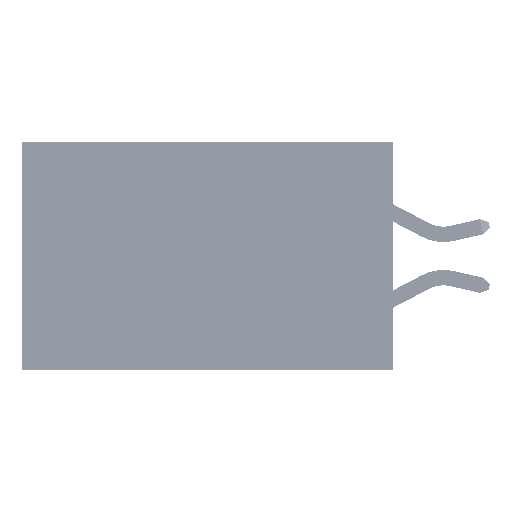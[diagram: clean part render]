
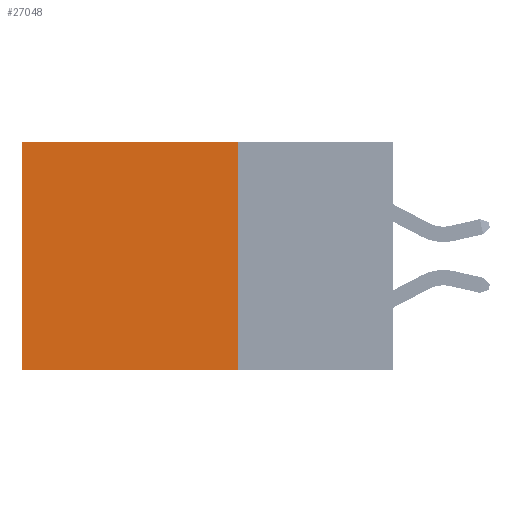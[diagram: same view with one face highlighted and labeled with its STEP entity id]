
A CAD part, left-side view. The second image highlights one B-rep face of the part: STEP entity #27048.
In plain terms, the highlighted planar face has unit normal (-1, 0, 0).
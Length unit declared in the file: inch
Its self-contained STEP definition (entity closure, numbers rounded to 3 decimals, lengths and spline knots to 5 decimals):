
#1830 = ORIENTED_EDGE ( 'NONE', *, *, #5780, .T. ) ;
#2251 = AXIS2_PLACEMENT_3D ( 'NONE', #22055, #33531, #18820 ) ;
#2702 = FACE_OUTER_BOUND ( 'NONE', #6475, .T. ) ;
#5780 = EDGE_CURVE ( 'NONE', #14651, #26979, #20097, .T. ) ;
#6475 = EDGE_LOOP ( 'NONE', ( #14346, #16748, #8131, #1830 ) ) ;
#8131 = ORIENTED_EDGE ( 'NONE', *, *, #28855, .F. ) ;
#9143 = VECTOR ( 'NONE', #19988, 39.37008 ) ;
#9574 = LINE ( 'NONE', #16689, #29916 ) ;
#12429 = VERTEX_POINT ( 'NONE', #32732 ) ;
#14346 = ORIENTED_EDGE ( 'NONE', *, *, #26588, .T. ) ;
#14651 = VERTEX_POINT ( 'NONE', #32349 ) ;
#15039 = CARTESIAN_POINT ( 'NONE',  ( 0.2875, 0.6, 0. ) ) ;
#16535 = VECTOR ( 'NONE', #17189, 39.37008 ) ;
#16689 = CARTESIAN_POINT ( 'NONE',  ( 0.2875, 0.25, -0.37 ) ) ;
#16748 = ORIENTED_EDGE ( 'NONE', *, *, #21354, .F. ) ;
#16850 = DIRECTION ( 'NONE',  ( 0., 1., 0. ) ) ;
#17189 = DIRECTION ( 'NONE',  ( 0., 0., -1. ) ) ;
#18820 = DIRECTION ( 'NONE',  ( 0., 0., -1. ) ) ;
#19988 = DIRECTION ( 'NONE',  ( 0., 0., -1. ) ) ;
#20097 = LINE ( 'NONE', #20265, #47301 ) ;
#20265 = CARTESIAN_POINT ( 'NONE',  ( 0.2875, 0.25, 0. ) ) ;
#21354 = EDGE_CURVE ( 'NONE', #12429, #30781, #9574, .T. ) ;
#22055 = CARTESIAN_POINT ( 'NONE',  ( 0.2875, 0.25, 0. ) ) ;
#23180 = DIRECTION ( 'NONE',  ( 0., 1., 0. ) ) ;
#26588 = EDGE_CURVE ( 'NONE', #26979, #30781, #41065, .T. ) ;
#26979 = VERTEX_POINT ( 'NONE', #15039 ) ;
#27048 = ADVANCED_FACE ( 'NONE', ( #2702 ), #40672, .F. ) ;
#28504 = CARTESIAN_POINT ( 'NONE',  ( 0.2875, 0.25, 0. ) ) ;
#28855 = EDGE_CURVE ( 'NONE', #14651, #12429, #37418, .T. ) ;
#29916 = VECTOR ( 'NONE', #16850, 39.37008 ) ;
#30781 = VERTEX_POINT ( 'NONE', #36061 ) ;
#32349 = CARTESIAN_POINT ( 'NONE',  ( 0.2875, 0.25, 0. ) ) ;
#32732 = CARTESIAN_POINT ( 'NONE',  ( 0.2875, 0.25, -0.37 ) ) ;
#33531 = DIRECTION ( 'NONE',  ( 1., 0., 0. ) ) ;
#36061 = CARTESIAN_POINT ( 'NONE',  ( 0.2875, 0.6, -0.37 ) ) ;
#37418 = LINE ( 'NONE', #28504, #16535 ) ;
#40672 = PLANE ( 'NONE',  #2251 ) ;
#41065 = LINE ( 'NONE', #42312, #9143 ) ;
#42312 = CARTESIAN_POINT ( 'NONE',  ( 0.2875, 0.6, 0. ) ) ;
#47301 = VECTOR ( 'NONE', #23180, 39.37008 ) ;
